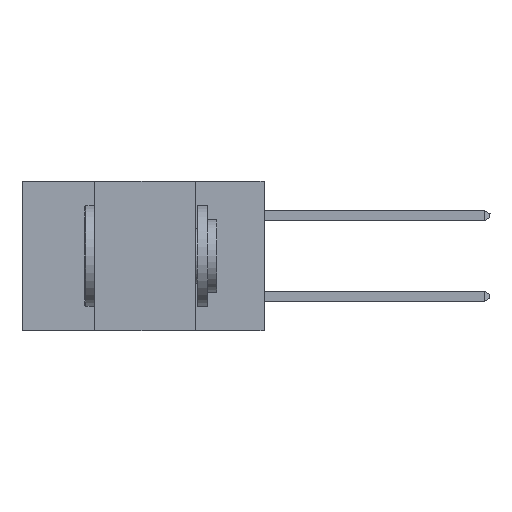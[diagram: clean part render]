
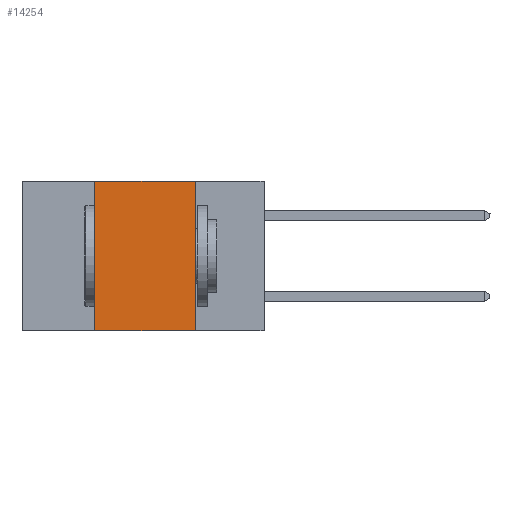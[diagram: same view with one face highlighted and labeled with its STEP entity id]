
A CAD part, left-side view. The second image highlights one B-rep face of the part: STEP entity #14254.
In plain terms, the highlighted planar face has unit normal (-1, 0, 0).
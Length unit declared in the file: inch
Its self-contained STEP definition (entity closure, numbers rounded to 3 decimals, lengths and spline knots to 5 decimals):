
#597 = CARTESIAN_POINT ( 'NONE',  ( 0., 0.42, 0. ) ) ;
#943 = LINE ( 'NONE', #13711, #6703 ) ;
#1205 = DIRECTION ( 'NONE',  ( 0., 0., -1. ) ) ;
#2039 = CARTESIAN_POINT ( 'NONE',  ( 0., 0.17, 0. ) ) ;
#2536 = VERTEX_POINT ( 'NONE', #20776 ) ;
#3196 = DIRECTION ( 'NONE',  ( 1., 0., 0. ) ) ;
#3980 = AXIS2_PLACEMENT_3D ( 'NONE', #13246, #3196, #1205 ) ;
#4312 = DIRECTION ( 'NONE',  ( 0., 0., 1. ) ) ;
#4376 = ORIENTED_EDGE ( 'NONE', *, *, #9838, .F. ) ;
#4880 = CARTESIAN_POINT ( 'NONE',  ( 0., 0.6, -0.37 ) ) ;
#5321 = LINE ( 'NONE', #2039, #17673 ) ;
#6643 = ORIENTED_EDGE ( 'NONE', *, *, #7935, .T. ) ;
#6703 = VECTOR ( 'NONE', #10360, 39.37008 ) ;
#7167 = DIRECTION ( 'NONE',  ( 0., 0., -1. ) ) ;
#7835 = LINE ( 'NONE', #4880, #16750 ) ;
#7935 = EDGE_CURVE ( 'NONE', #11240, #14271, #7835, .T. ) ;
#8142 = VERTEX_POINT ( 'NONE', #597 ) ;
#8400 = ORIENTED_EDGE ( 'NONE', *, *, #16033, .F. ) ;
#8641 = CARTESIAN_POINT ( 'NONE',  ( 0., 0.42, -0.37 ) ) ;
#9193 = EDGE_CURVE ( 'NONE', #8142, #2536, #943, .T. ) ;
#9199 = CARTESIAN_POINT ( 'NONE',  ( 0., 0.42, 0. ) ) ;
#9588 = LINE ( 'NONE', #9199, #11158 ) ;
#9767 = EDGE_LOOP ( 'NONE', ( #8400, #12938, #4376, #6643 ) ) ;
#9838 = EDGE_CURVE ( 'NONE', #11240, #8142, #9588, .T. ) ;
#10131 = DIRECTION ( 'NONE',  ( 0., -1., 0. ) ) ;
#10360 = DIRECTION ( 'NONE',  ( 0., -1., 0. ) ) ;
#11158 = VECTOR ( 'NONE', #4312, 39.37008 ) ;
#11240 = VERTEX_POINT ( 'NONE', #8641 ) ;
#12533 = FACE_OUTER_BOUND ( 'NONE', #9767, .T. ) ;
#12938 = ORIENTED_EDGE ( 'NONE', *, *, #9193, .F. ) ;
#13246 = CARTESIAN_POINT ( 'NONE',  ( 0., 0.6, 0. ) ) ;
#13711 = CARTESIAN_POINT ( 'NONE',  ( 0., 0.6, 0. ) ) ;
#14254 = ADVANCED_FACE ( 'NONE', ( #12533 ), #19811, .F. ) ;
#14271 = VERTEX_POINT ( 'NONE', #21397 ) ;
#16033 = EDGE_CURVE ( 'NONE', #2536, #14271, #5321, .T. ) ;
#16750 = VECTOR ( 'NONE', #10131, 39.37008 ) ;
#17673 = VECTOR ( 'NONE', #7167, 39.37008 ) ;
#19811 = PLANE ( 'NONE',  #3980 ) ;
#20776 = CARTESIAN_POINT ( 'NONE',  ( 0., 0.17, 0. ) ) ;
#21397 = CARTESIAN_POINT ( 'NONE',  ( 0., 0.17, -0.37 ) ) ;
